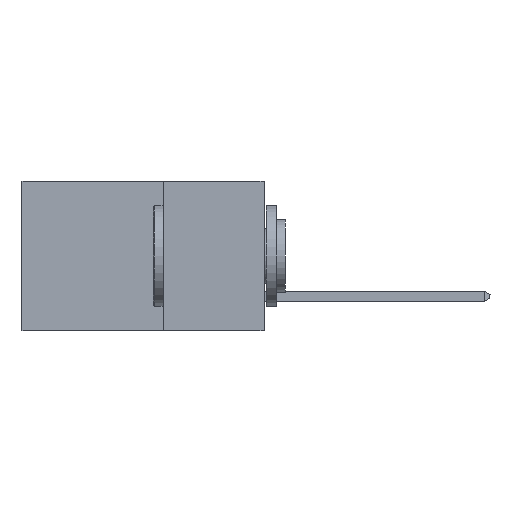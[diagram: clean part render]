
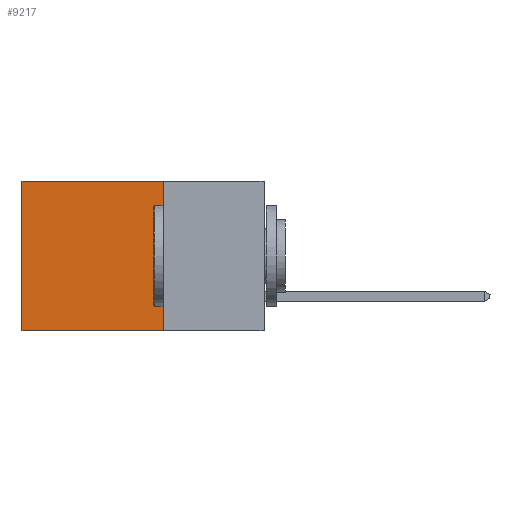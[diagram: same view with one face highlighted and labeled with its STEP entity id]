
A CAD part, left-side view. The second image highlights one B-rep face of the part: STEP entity #9217.
In plain terms, the highlighted planar face has unit normal (-1, 0, 0).
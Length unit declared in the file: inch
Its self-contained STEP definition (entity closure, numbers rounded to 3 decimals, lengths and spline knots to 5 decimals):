
#130 = ORIENTED_EDGE ( 'NONE', *, *, #2934, .T. ) ;
#303 = VECTOR ( 'NONE', #13810, 39.37008 ) ;
#682 = VERTEX_POINT ( 'NONE', #4212 ) ;
#956 = DIRECTION ( 'NONE',  ( 0., 0., -1. ) ) ;
#983 = ORIENTED_EDGE ( 'NONE', *, *, #9750, .F. ) ;
#1031 = ORIENTED_EDGE ( 'NONE', *, *, #3114, .T. ) ;
#1215 = CARTESIAN_POINT ( 'NONE',  ( 0.298, 0.25, 0. ) ) ;
#1840 = CARTESIAN_POINT ( 'NONE',  ( 0.298, 0.6, 0. ) ) ;
#2312 = VECTOR ( 'NONE', #11778, 39.37008 ) ;
#2555 = VECTOR ( 'NONE', #5475, 39.37008 ) ;
#2934 = EDGE_CURVE ( 'NONE', #3969, #4727, #13448, .T. ) ;
#3066 = CARTESIAN_POINT ( 'NONE',  ( 0.298, 0.25, 0. ) ) ;
#3114 = EDGE_CURVE ( 'NONE', #682, #3969, #9863, .T. ) ;
#3391 = CARTESIAN_POINT ( 'NONE',  ( 0.298, 0.25, -0.37 ) ) ;
#3969 = VERTEX_POINT ( 'NONE', #12835 ) ;
#4035 = AXIS2_PLACEMENT_3D ( 'NONE', #12522, #13645, #7122 ) ;
#4212 = CARTESIAN_POINT ( 'NONE',  ( 0.298, 0.25, 0. ) ) ;
#4534 = EDGE_CURVE ( 'NONE', #11466, #4727, #13722, .T. ) ;
#4727 = VERTEX_POINT ( 'NONE', #13626 ) ;
#5475 = DIRECTION ( 'NONE',  ( 0., 0., -1. ) ) ;
#6642 = ORIENTED_EDGE ( 'NONE', *, *, #4534, .F. ) ;
#7122 = DIRECTION ( 'NONE',  ( 0., 0., -1. ) ) ;
#7396 = CARTESIAN_POINT ( 'NONE',  ( 0.298, 0.25, -0.37 ) ) ;
#8280 = PLANE ( 'NONE',  #4035 ) ;
#9072 = VECTOR ( 'NONE', #956, 39.37008 ) ;
#9217 = ADVANCED_FACE ( 'NONE', ( #11639 ), #8280, .F. ) ;
#9750 = EDGE_CURVE ( 'NONE', #682, #11466, #12954, .T. ) ;
#9863 = LINE ( 'NONE', #3066, #303 ) ;
#11466 = VERTEX_POINT ( 'NONE', #3391 ) ;
#11639 = FACE_OUTER_BOUND ( 'NONE', #13337, .T. ) ;
#11778 = DIRECTION ( 'NONE',  ( 0., 1., 0. ) ) ;
#12522 = CARTESIAN_POINT ( 'NONE',  ( 0.298, 0.25, 0. ) ) ;
#12835 = CARTESIAN_POINT ( 'NONE',  ( 0.298, 0.6, 0. ) ) ;
#12954 = LINE ( 'NONE', #1215, #9072 ) ;
#13337 = EDGE_LOOP ( 'NONE', ( #130, #6642, #983, #1031 ) ) ;
#13448 = LINE ( 'NONE', #1840, #2555 ) ;
#13626 = CARTESIAN_POINT ( 'NONE',  ( 0.298, 0.6, -0.37 ) ) ;
#13645 = DIRECTION ( 'NONE',  ( 1., 0., 0. ) ) ;
#13722 = LINE ( 'NONE', #7396, #2312 ) ;
#13810 = DIRECTION ( 'NONE',  ( 0., 1., 0. ) ) ;
